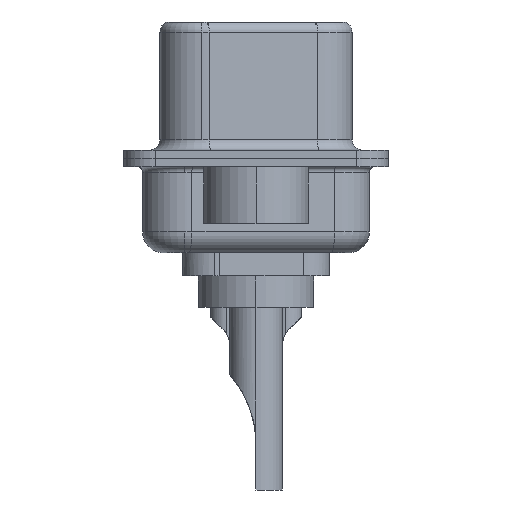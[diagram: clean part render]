
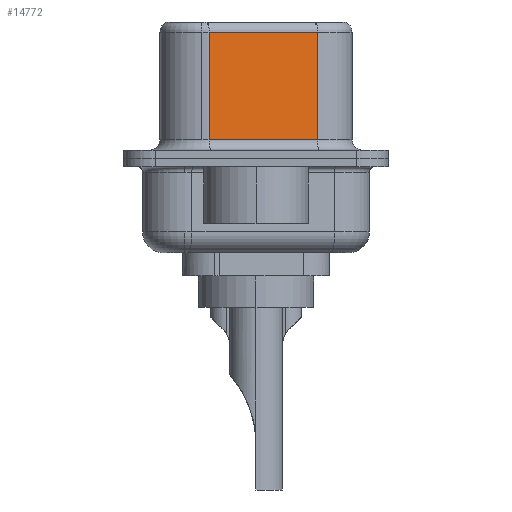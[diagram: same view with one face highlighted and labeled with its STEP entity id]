
A CAD part, left-side view. The second image highlights one B-rep face of the part: STEP entity #14772.
In plain terms, the highlighted planar face has unit normal (-0.985, -0.174, 0).
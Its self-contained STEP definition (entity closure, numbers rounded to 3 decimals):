
#152 = ORIENTED_EDGE ( 'NONE', *, *, #20065, .T. ) ;
#688 = VERTEX_POINT ( 'NONE', #13694 ) ;
#1493 = FACE_OUTER_BOUND ( 'NONE', #23155, .T. ) ;
#1630 = DIRECTION ( 'NONE',  ( 0., 0., -1. ) ) ;
#3478 = CARTESIAN_POINT ( 'NONE',  ( 4.58, -2.927, 0.9 ) ) ;
#3789 = DIRECTION ( 'NONE',  ( 0.985, 0.174, 0. ) ) ;
#3851 = DIRECTION ( 'NONE',  ( -0.174, 0.985, 0. ) ) ;
#4731 = LINE ( 'NONE', #11404, #24285 ) ;
#6926 = CARTESIAN_POINT ( 'NONE',  ( 4.58, -2.927, 6.02 ) ) ;
#7129 = VECTOR ( 'NONE', #20602, 1000. ) ;
#8482 = VECTOR ( 'NONE', #18957, 1000. ) ;
#9190 = EDGE_CURVE ( 'NONE', #13322, #20187, #4731, .T. ) ;
#11015 = VERTEX_POINT ( 'NONE', #18973 ) ;
#11404 = CARTESIAN_POINT ( 'NONE',  ( 4.58, -2.927, 6.02 ) ) ;
#12174 = LINE ( 'NONE', #3478, #7129 ) ;
#12758 = ORIENTED_EDGE ( 'NONE', *, *, #22637, .T. ) ;
#13322 = VERTEX_POINT ( 'NONE', #6926 ) ;
#13694 = CARTESIAN_POINT ( 'NONE',  ( 4.58, -2.927, 0.9 ) ) ;
#14078 = AXIS2_PLACEMENT_3D ( 'NONE', #14744, #3789, #17021 ) ;
#14744 = CARTESIAN_POINT ( 'NONE',  ( 4.58, -2.927, 6.52 ) ) ;
#14772 = ADVANCED_FACE ( 'NONE', ( #1493 ), #15156, .F. ) ;
#15156 = PLANE ( 'NONE',  #14078 ) ;
#17021 = DIRECTION ( 'NONE',  ( -0.174, 0.985, 0. ) ) ;
#17061 = CARTESIAN_POINT ( 'NONE',  ( 4.58, -2.927, 6.52 ) ) ;
#18717 = LINE ( 'NONE', #24357, #24388 ) ;
#18957 = DIRECTION ( 'NONE',  ( 0., 0., -1. ) ) ;
#18973 = CARTESIAN_POINT ( 'NONE',  ( 3.67, 2.233, 0.9 ) ) ;
#19021 = ORIENTED_EDGE ( 'NONE', *, *, #24240, .F. ) ;
#20065 = EDGE_CURVE ( 'NONE', #20187, #11015, #18717, .T. ) ;
#20187 = VERTEX_POINT ( 'NONE', #22666 ) ;
#20602 = DIRECTION ( 'NONE',  ( 0.174, -0.985, 0. ) ) ;
#22637 = EDGE_CURVE ( 'NONE', #11015, #688, #12174, .T. ) ;
#22666 = CARTESIAN_POINT ( 'NONE',  ( 3.67, 2.233, 6.02 ) ) ;
#23155 = EDGE_LOOP ( 'NONE', ( #19021, #23244, #152, #12758 ) ) ;
#23244 = ORIENTED_EDGE ( 'NONE', *, *, #9190, .T. ) ;
#23594 = LINE ( 'NONE', #17061, #8482 ) ;
#24240 = EDGE_CURVE ( 'NONE', #13322, #688, #23594, .T. ) ;
#24285 = VECTOR ( 'NONE', #3851, 1000. ) ;
#24357 = CARTESIAN_POINT ( 'NONE',  ( 3.67, 2.233, 6.52 ) ) ;
#24388 = VECTOR ( 'NONE', #1630, 1000. ) ;
